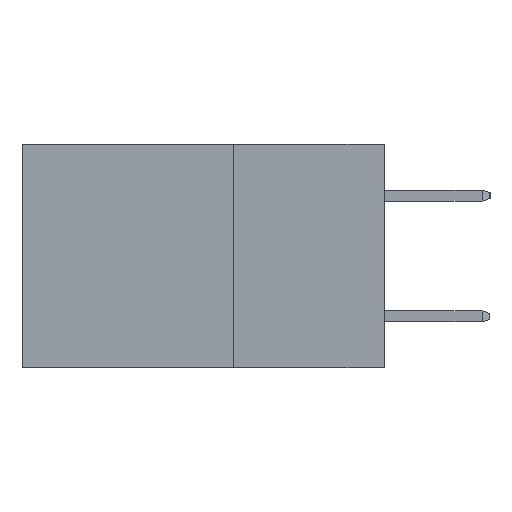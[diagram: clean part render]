
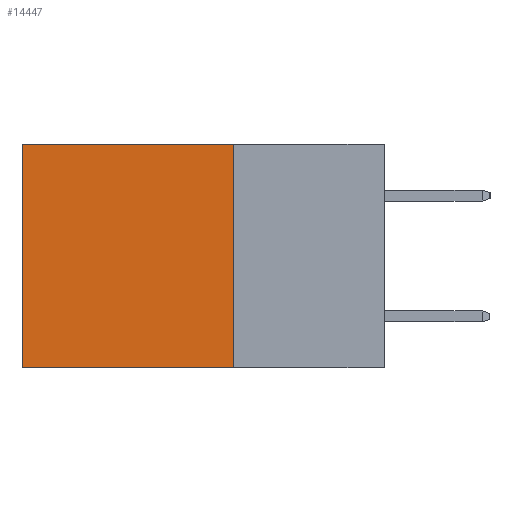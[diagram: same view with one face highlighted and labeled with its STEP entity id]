
A CAD part, left-side view. The second image highlights one B-rep face of the part: STEP entity #14447.
In plain terms, the highlighted planar face has unit normal (-1, 0, 0).
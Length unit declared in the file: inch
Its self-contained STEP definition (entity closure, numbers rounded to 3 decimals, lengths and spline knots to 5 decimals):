
#454 = EDGE_CURVE ( 'NONE', #2117, #13247, #5212, .T. ) ;
#1178 = PLANE ( 'NONE',  #4141 ) ;
#1179 = CARTESIAN_POINT ( 'NONE',  ( 0.298, 0.6, -0.37 ) ) ;
#2117 = VERTEX_POINT ( 'NONE', #9561 ) ;
#2377 = DIRECTION ( 'NONE',  ( 0., 0., -1. ) ) ;
#2500 = VECTOR ( 'NONE', #8816, 39.37008 ) ;
#2667 = EDGE_LOOP ( 'NONE', ( #10811, #7291, #6189, #3121 ) ) ;
#2968 = DIRECTION ( 'NONE',  ( 0., 1., 0. ) ) ;
#3021 = CARTESIAN_POINT ( 'NONE',  ( 0.298, 0.25, 0. ) ) ;
#3121 = ORIENTED_EDGE ( 'NONE', *, *, #7080, .T. ) ;
#3815 = VECTOR ( 'NONE', #2968, 39.37008 ) ;
#3993 = DIRECTION ( 'NONE',  ( 0., 1., 0. ) ) ;
#4043 = CARTESIAN_POINT ( 'NONE',  ( 0.298, 0.6, 0. ) ) ;
#4094 = EDGE_CURVE ( 'NONE', #12399, #10649, #5658, .T. ) ;
#4141 = AXIS2_PLACEMENT_3D ( 'NONE', #5889, #9318, #2377 ) ;
#5212 = LINE ( 'NONE', #4043, #7206 ) ;
#5658 = LINE ( 'NONE', #10854, #2500 ) ;
#5889 = CARTESIAN_POINT ( 'NONE',  ( 0.298, 0.25, 0. ) ) ;
#6189 = ORIENTED_EDGE ( 'NONE', *, *, #4094, .F. ) ;
#7044 = LINE ( 'NONE', #10765, #10017 ) ;
#7080 = EDGE_CURVE ( 'NONE', #12399, #2117, #10223, .T. ) ;
#7206 = VECTOR ( 'NONE', #11148, 39.37008 ) ;
#7291 = ORIENTED_EDGE ( 'NONE', *, *, #12785, .F. ) ;
#7888 = CARTESIAN_POINT ( 'NONE',  ( 0.298, 0.25, -0.37 ) ) ;
#8816 = DIRECTION ( 'NONE',  ( 0., 0., -1. ) ) ;
#9318 = DIRECTION ( 'NONE',  ( 1., 0., 0. ) ) ;
#9561 = CARTESIAN_POINT ( 'NONE',  ( 0.298, 0.6, 0. ) ) ;
#10017 = VECTOR ( 'NONE', #3993, 39.37008 ) ;
#10223 = LINE ( 'NONE', #3021, #3815 ) ;
#10649 = VERTEX_POINT ( 'NONE', #7888 ) ;
#10765 = CARTESIAN_POINT ( 'NONE',  ( 0.298, 0.25, -0.37 ) ) ;
#10811 = ORIENTED_EDGE ( 'NONE', *, *, #454, .T. ) ;
#10854 = CARTESIAN_POINT ( 'NONE',  ( 0.298, 0.25, 0. ) ) ;
#11148 = DIRECTION ( 'NONE',  ( 0., 0., -1. ) ) ;
#12399 = VERTEX_POINT ( 'NONE', #14324 ) ;
#12785 = EDGE_CURVE ( 'NONE', #10649, #13247, #7044, .T. ) ;
#13114 = FACE_OUTER_BOUND ( 'NONE', #2667, .T. ) ;
#13247 = VERTEX_POINT ( 'NONE', #1179 ) ;
#14324 = CARTESIAN_POINT ( 'NONE',  ( 0.298, 0.25, 0. ) ) ;
#14447 = ADVANCED_FACE ( 'NONE', ( #13114 ), #1178, .F. ) ;
